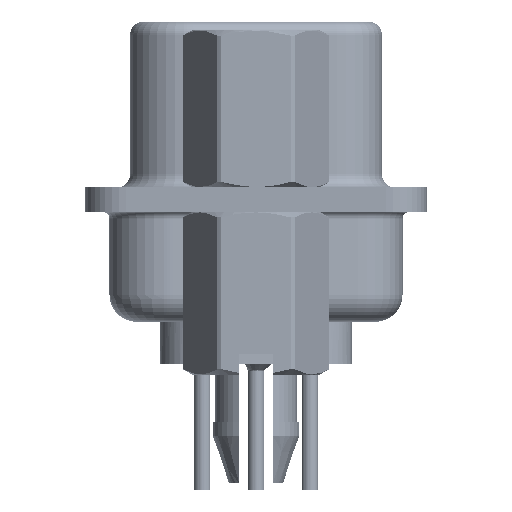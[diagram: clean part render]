
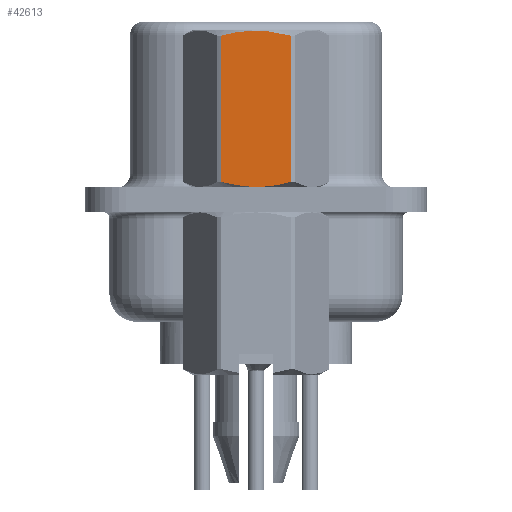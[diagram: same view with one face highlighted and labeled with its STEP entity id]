
A CAD part, left-side view. The second image highlights one B-rep face of the part: STEP entity #42613.
In plain terms, the highlighted planar face has unit normal (-1, 0, 0).
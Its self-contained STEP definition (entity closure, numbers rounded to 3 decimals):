
#584 = CARTESIAN_POINT ( 'NONE',  ( -2.381, 1.375, -3.75 ) ) ;
#1184 = CARTESIAN_POINT ( 'NONE',  ( -2.381, 1.065, 0.596 ) ) ;
#1844 = CARTESIAN_POINT ( 'NONE',  ( -2.381, -1.066, 0.596 ) ) ;
#2437 = CARTESIAN_POINT ( 'NONE',  ( -2.381, 0.853, 6.151 ) ) ;
#2595 = VECTOR ( 'NONE', #23351, 1000. ) ;
#2850 = VECTOR ( 'NONE', #14789, 1000. ) ;
#4845 = CARTESIAN_POINT ( 'NONE',  ( -2.381, -0.215, 0.468 ) ) ;
#7710 = DIRECTION ( 'NONE',  ( 0., -1., 0. ) ) ;
#7936 = CARTESIAN_POINT ( 'NONE',  ( -2.381, 1.273, 3.792 ) ) ;
#9102 = CARTESIAN_POINT ( 'NONE',  ( -2.381, -1.066, 6.104 ) ) ;
#10451 = FACE_OUTER_BOUND ( 'NONE', #13162, .T. ) ;
#10600 = EDGE_CURVE ( 'NONE', #44437, #19915, #11110, .T. ) ;
#11110 = B_SPLINE_CURVE_WITH_KNOTS ( 'NONE', 3,
 ( #12737, #9102, #40919, #33833, #15750, #36595, #19411, #2437, #40250, #33611 ),
 .UNSPECIFIED., .F., .F.,
 ( 4, 2, 2, 2, 4 ),
 ( 0.001, 0.002, 0.002, 0.003, 0.004 ),
 .UNSPECIFIED. ) ;
#11709 = CARTESIAN_POINT ( 'NONE',  ( -2.381, 0.215, 0.468 ) ) ;
#11963 = CARTESIAN_POINT ( 'NONE',  ( -2.381, 1.273, 0.652 ) ) ;
#12737 = CARTESIAN_POINT ( 'NONE',  ( -2.381, -1.273, 6.048 ) ) ;
#12935 = ORIENTED_EDGE ( 'NONE', *, *, #37805, .T. ) ;
#13162 = EDGE_LOOP ( 'NONE', ( #40340, #12935, #21158, #20149 ) ) ;
#13872 = DIRECTION ( 'NONE',  ( -1., 0., 0. ) ) ;
#14789 = DIRECTION ( 'NONE',  ( 0., 0., -1. ) ) ;
#15080 = CARTESIAN_POINT ( 'NONE',  ( -2.381, 1.273, 6.048 ) ) ;
#15160 = CARTESIAN_POINT ( 'NONE',  ( -2.381, 0.853, 0.549 ) ) ;
#15218 = CARTESIAN_POINT ( 'NONE',  ( -2.381, -1.273, 6.048 ) ) ;
#15750 = CARTESIAN_POINT ( 'NONE',  ( -2.381, -0.215, 6.232 ) ) ;
#16471 = CARTESIAN_POINT ( 'NONE',  ( -2.381, -1.273, 3.792 ) ) ;
#19020 = VERTEX_POINT ( 'NONE', #11963 ) ;
#19411 = CARTESIAN_POINT ( 'NONE',  ( -2.381, 0.428, 6.215 ) ) ;
#19670 = AXIS2_PLACEMENT_3D ( 'NONE', #584, #13872, #7710 ) ;
#19688 = LINE ( 'NONE', #16471, #2595 ) ;
#19915 = VERTEX_POINT ( 'NONE', #15080 ) ;
#20149 = ORIENTED_EDGE ( 'NONE', *, *, #42856, .T. ) ;
#21007 = PLANE ( 'NONE',  #19670 ) ;
#21158 = ORIENTED_EDGE ( 'NONE', *, *, #10600, .T. ) ;
#21639 = EDGE_CURVE ( 'NONE', #19020, #38455, #31115, .T. ) ;
#22723 = CARTESIAN_POINT ( 'NONE',  ( -2.381, -1.273, 0.652 ) ) ;
#23351 = DIRECTION ( 'NONE',  ( 0., 0., 1. ) ) ;
#25698 = CARTESIAN_POINT ( 'NONE',  ( -2.381, -0.432, 0.485 ) ) ;
#29364 = CARTESIAN_POINT ( 'NONE',  ( -2.381, 1.273, 0.652 ) ) ;
#31115 = B_SPLINE_CURVE_WITH_KNOTS ( 'NONE', 3,
 ( #29364, #1184, #15160, #43094, #11709, #4845, #25698, #33245, #1844, #22723 ),
 .UNSPECIFIED., .F., .F.,
 ( 4, 2, 2, 2, 4 ),
 ( 0.003, 0.003, 0.004, 0.004, 0.005 ),
 .UNSPECIFIED. ) ;
#33245 = CARTESIAN_POINT ( 'NONE',  ( -2.381, -0.858, 0.55 ) ) ;
#33611 = CARTESIAN_POINT ( 'NONE',  ( -2.381, 1.273, 6.048 ) ) ;
#33833 = CARTESIAN_POINT ( 'NONE',  ( -2.381, -0.432, 6.215 ) ) ;
#36548 = LINE ( 'NONE', #7936, #2850 ) ;
#36595 = CARTESIAN_POINT ( 'NONE',  ( -2.381, 0.215, 6.232 ) ) ;
#37805 = EDGE_CURVE ( 'NONE', #38455, #44437, #19688, .T. ) ;
#38455 = VERTEX_POINT ( 'NONE', #42196 ) ;
#40250 = CARTESIAN_POINT ( 'NONE',  ( -2.381, 1.065, 6.104 ) ) ;
#40340 = ORIENTED_EDGE ( 'NONE', *, *, #21639, .T. ) ;
#40919 = CARTESIAN_POINT ( 'NONE',  ( -2.381, -0.858, 6.15 ) ) ;
#42196 = CARTESIAN_POINT ( 'NONE',  ( -2.381, -1.273, 0.652 ) ) ;
#42613 = ADVANCED_FACE ( 'NONE', ( #10451 ), #21007, .T. ) ;
#42856 = EDGE_CURVE ( 'NONE', #19915, #19020, #36548, .T. ) ;
#43094 = CARTESIAN_POINT ( 'NONE',  ( -2.381, 0.428, 0.485 ) ) ;
#44437 = VERTEX_POINT ( 'NONE', #15218 ) ;
